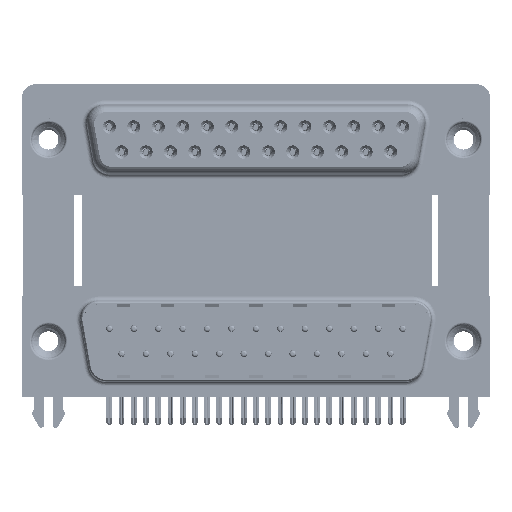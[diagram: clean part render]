
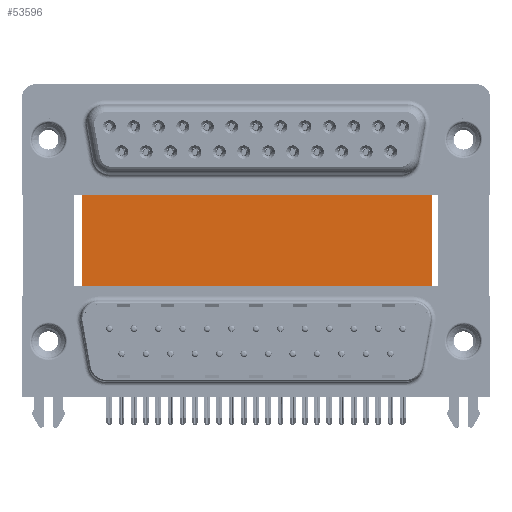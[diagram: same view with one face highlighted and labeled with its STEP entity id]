
A CAD part, top view. The second image highlights one B-rep face of the part: STEP entity #53596.
In plain terms, the highlighted planar face has unit normal (0, 0, 1).
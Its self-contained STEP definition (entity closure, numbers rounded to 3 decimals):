
#317 = VECTOR ( 'NONE', #51060, 1000. ) ;
#371 = LINE ( 'NONE', #53862, #12931 ) ;
#4181 = FACE_OUTER_BOUND ( 'NONE', #15166, .T. ) ;
#4755 = PLANE ( 'NONE',  #4837 ) ;
#4837 = AXIS2_PLACEMENT_3D ( 'NONE', #48923, #49515, #27457 ) ;
#7195 = ORIENTED_EDGE ( 'NONE', *, *, #41993, .F. ) ;
#9711 = VERTEX_POINT ( 'NONE', #23247 ) ;
#10193 = CARTESIAN_POINT ( 'NONE',  ( 3.79, -3.735, -12. ) ) ;
#12091 = EDGE_CURVE ( 'NONE', #40923, #30225, #371, .T. ) ;
#12931 = VECTOR ( 'NONE', #31783, 1000. ) ;
#14998 = EDGE_CURVE ( 'NONE', #30225, #15679, #33264, .T. ) ;
#15166 = EDGE_LOOP ( 'NONE', ( #42286, #7195, #52286, #22750 ) ) ;
#15679 = VERTEX_POINT ( 'NONE', #19342 ) ;
#17477 = EDGE_CURVE ( 'NONE', #40923, #9711, #38105, .T. ) ;
#19342 = CARTESIAN_POINT ( 'NONE',  ( 43.43, -3.735, -12. ) ) ;
#21488 = VECTOR ( 'NONE', #37903, 1000. ) ;
#22750 = ORIENTED_EDGE ( 'NONE', *, *, #12091, .T. ) ;
#23247 = CARTESIAN_POINT ( 'NONE',  ( 43.43, 16.585, -12. ) ) ;
#23910 = CARTESIAN_POINT ( 'NONE',  ( 3.79, 16.585, -12. ) ) ;
#27457 = DIRECTION ( 'NONE',  ( -1., 0., 0. ) ) ;
#30225 = VERTEX_POINT ( 'NONE', #10193 ) ;
#31783 = DIRECTION ( 'NONE',  ( 0., -1., 0. ) ) ;
#33264 = LINE ( 'NONE', #55946, #21488 ) ;
#37819 = CARTESIAN_POINT ( 'NONE',  ( 3.79, 16.585, -12. ) ) ;
#37903 = DIRECTION ( 'NONE',  ( 1., 0., 0. ) ) ;
#38105 = LINE ( 'NONE', #23910, #56395 ) ;
#38552 = LINE ( 'NONE', #51930, #317 ) ;
#40923 = VERTEX_POINT ( 'NONE', #37819 ) ;
#41993 = EDGE_CURVE ( 'NONE', #9711, #15679, #38552, .T. ) ;
#42286 = ORIENTED_EDGE ( 'NONE', *, *, #14998, .T. ) ;
#48923 = CARTESIAN_POINT ( 'NONE',  ( 3.79, 16.585, -12. ) ) ;
#49515 = DIRECTION ( 'NONE',  ( 0., 0., -1. ) ) ;
#51060 = DIRECTION ( 'NONE',  ( 0., -1., 0. ) ) ;
#51930 = CARTESIAN_POINT ( 'NONE',  ( 43.43, 16.585, -12. ) ) ;
#52286 = ORIENTED_EDGE ( 'NONE', *, *, #17477, .F. ) ;
#53596 = ADVANCED_FACE ( 'NONE', ( #4181 ), #4755, .F. ) ;
#53862 = CARTESIAN_POINT ( 'NONE',  ( 3.79, 16.585, -12. ) ) ;
#55864 = DIRECTION ( 'NONE',  ( 1., 0., 0. ) ) ;
#55946 = CARTESIAN_POINT ( 'NONE',  ( 3.79, -3.735, -12. ) ) ;
#56395 = VECTOR ( 'NONE', #55864, 1000. ) ;
